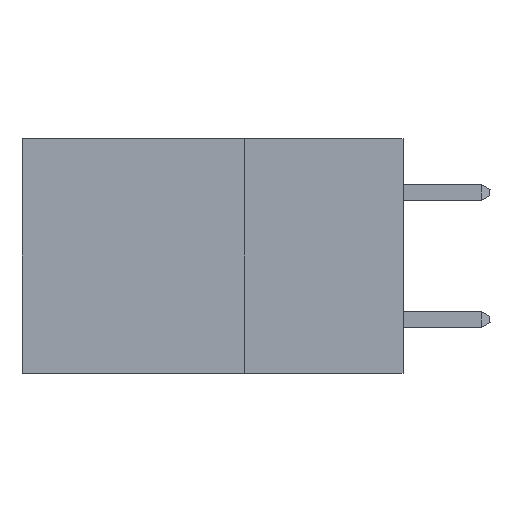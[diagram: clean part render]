
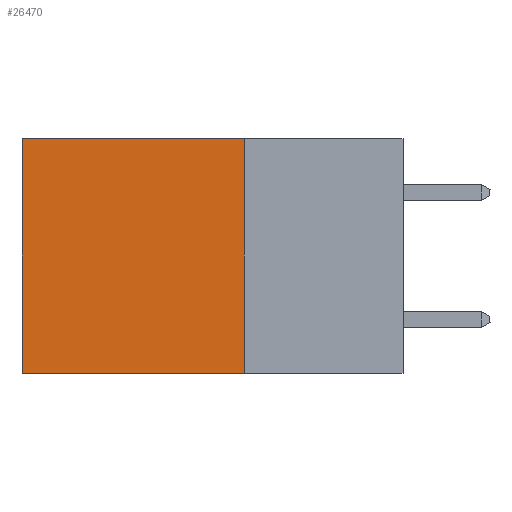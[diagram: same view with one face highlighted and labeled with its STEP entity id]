
A CAD part, left-side view. The second image highlights one B-rep face of the part: STEP entity #26470.
In plain terms, the highlighted planar face has unit normal (-1, 0, 0).
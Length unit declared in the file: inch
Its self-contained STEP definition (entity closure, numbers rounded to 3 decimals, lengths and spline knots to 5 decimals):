
#138 = VECTOR ( 'NONE', #23981, 39.37008 ) ;
#1018 = VECTOR ( 'NONE', #30672, 39.37008 ) ;
#2231 = LINE ( 'NONE', #17632, #1018 ) ;
#3259 = ORIENTED_EDGE ( 'NONE', *, *, #21961, .T. ) ;
#4755 = CARTESIAN_POINT ( 'NONE',  ( 0.2875, 0.6, 0. ) ) ;
#7380 = DIRECTION ( 'NONE',  ( 0., 1., 0. ) ) ;
#9688 = ORIENTED_EDGE ( 'NONE', *, *, #14404, .F. ) ;
#9755 = DIRECTION ( 'NONE',  ( 0., 0., -1. ) ) ;
#11839 = DIRECTION ( 'NONE',  ( 0., 0., -1. ) ) ;
#12339 = VERTEX_POINT ( 'NONE', #15017 ) ;
#13080 = LINE ( 'NONE', #22396, #30100 ) ;
#13301 = CARTESIAN_POINT ( 'NONE',  ( 0.2875, 0.25, 0. ) ) ;
#14404 = EDGE_CURVE ( 'NONE', #33860, #12339, #19218, .T. ) ;
#14894 = CARTESIAN_POINT ( 'NONE',  ( 0.2875, 0.25, 0. ) ) ;
#15017 = CARTESIAN_POINT ( 'NONE',  ( 0.2875, 0.25, -0.37 ) ) ;
#15553 = CARTESIAN_POINT ( 'NONE',  ( 0.2875, 0.25, 0. ) ) ;
#15927 = AXIS2_PLACEMENT_3D ( 'NONE', #25771, #30974, #9755 ) ;
#16196 = EDGE_CURVE ( 'NONE', #24125, #24626, #13080, .T. ) ;
#17548 = ORIENTED_EDGE ( 'NONE', *, *, #16196, .T. ) ;
#17632 = CARTESIAN_POINT ( 'NONE',  ( 0.2875, 0.25, -0.37 ) ) ;
#17726 = EDGE_LOOP ( 'NONE', ( #17548, #18941, #9688, #3259 ) ) ;
#18941 = ORIENTED_EDGE ( 'NONE', *, *, #33806, .F. ) ;
#19218 = LINE ( 'NONE', #13301, #138 ) ;
#21858 = FACE_OUTER_BOUND ( 'NONE', #17726, .T. ) ;
#21961 = EDGE_CURVE ( 'NONE', #33860, #24125, #24143, .T. ) ;
#22396 = CARTESIAN_POINT ( 'NONE',  ( 0.2875, 0.6, 0. ) ) ;
#23981 = DIRECTION ( 'NONE',  ( 0., 0., -1. ) ) ;
#24125 = VERTEX_POINT ( 'NONE', #4755 ) ;
#24143 = LINE ( 'NONE', #14894, #29145 ) ;
#24626 = VERTEX_POINT ( 'NONE', #30896 ) ;
#25771 = CARTESIAN_POINT ( 'NONE',  ( 0.2875, 0.25, 0. ) ) ;
#26470 = ADVANCED_FACE ( 'NONE', ( #21858 ), #33736, .F. ) ;
#29145 = VECTOR ( 'NONE', #7380, 39.37008 ) ;
#30100 = VECTOR ( 'NONE', #11839, 39.37008 ) ;
#30672 = DIRECTION ( 'NONE',  ( 0., 1., 0. ) ) ;
#30896 = CARTESIAN_POINT ( 'NONE',  ( 0.2875, 0.6, -0.37 ) ) ;
#30974 = DIRECTION ( 'NONE',  ( 1., 0., 0. ) ) ;
#33736 = PLANE ( 'NONE',  #15927 ) ;
#33806 = EDGE_CURVE ( 'NONE', #12339, #24626, #2231, .T. ) ;
#33860 = VERTEX_POINT ( 'NONE', #15553 ) ;
